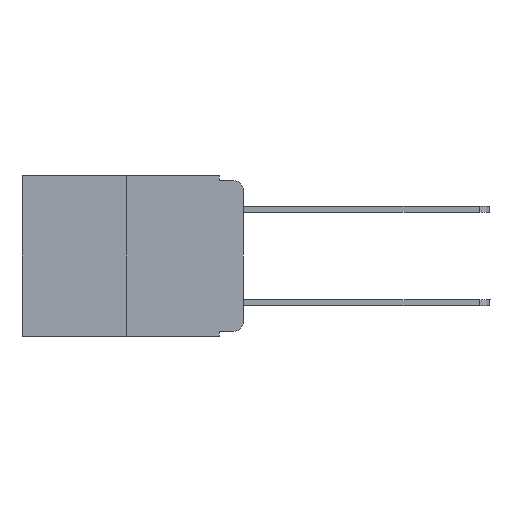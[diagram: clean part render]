
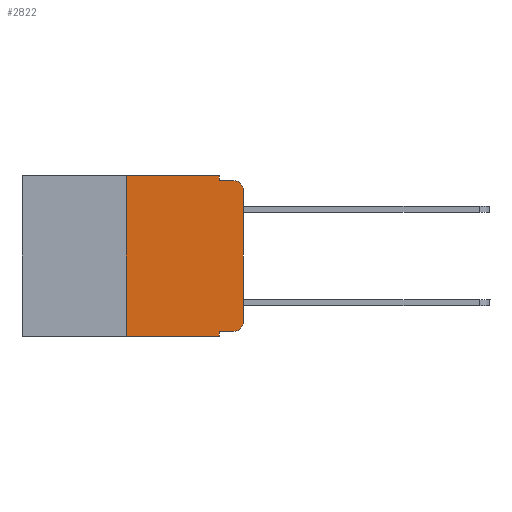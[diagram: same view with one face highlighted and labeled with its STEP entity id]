
A CAD part, left-side view. The second image highlights one B-rep face of the part: STEP entity #2822.
In plain terms, the highlighted planar face has unit normal (-1, 0, 0).
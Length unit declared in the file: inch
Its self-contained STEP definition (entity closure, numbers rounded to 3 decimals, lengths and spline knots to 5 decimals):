
#67 = LINE ( 'NONE', #15647, #533 ) ;
#316 = CARTESIAN_POINT ( 'NONE',  ( 0., 0.473, 0. ) ) ;
#466 = VECTOR ( 'NONE', #7113, 39.37008 ) ;
#524 = CARTESIAN_POINT ( 'NONE',  ( 0., 0.473, 0. ) ) ;
#533 = VECTOR ( 'NONE', #4068, 39.37008 ) ;
#613 = VECTOR ( 'NONE', #11572, 39.37008 ) ;
#622 = LINE ( 'NONE', #12232, #9896 ) ;
#713 = ORIENTED_EDGE ( 'NONE', *, *, #8931, .F. ) ;
#740 = ORIENTED_EDGE ( 'NONE', *, *, #4380, .T. ) ;
#883 = CARTESIAN_POINT ( 'NONE',  ( 0., 0.25, -0.343 ) ) ;
#1070 = CIRCLE ( 'NONE', #5091, 0.02 ) ;
#1348 = EDGE_CURVE ( 'NONE', #3318, #15145, #14514, .T. ) ;
#1510 = VERTEX_POINT ( 'NONE', #8373 ) ;
#2126 = VERTEX_POINT ( 'NONE', #2161 ) ;
#2161 = CARTESIAN_POINT ( 'NONE',  ( 0., 0., -0.313 ) ) ;
#2480 = EDGE_CURVE ( 'NONE', #13575, #7105, #11095, .T. ) ;
#2576 = DIRECTION ( 'NONE',  ( 0., 0., -1. ) ) ;
#2800 = CARTESIAN_POINT ( 'NONE',  ( 0., 0., 0. ) ) ;
#2822 = ADVANCED_FACE ( 'NONE', ( #15793 ), #3281, .F. ) ;
#3091 = DIRECTION ( 'NONE',  ( 0., 0., -1. ) ) ;
#3263 = ORIENTED_EDGE ( 'NONE', *, *, #14166, .F. ) ;
#3281 = PLANE ( 'NONE',  #10324 ) ;
#3283 = DIRECTION ( 'NONE',  ( 0., 0., -1. ) ) ;
#3318 = VERTEX_POINT ( 'NONE', #14580 ) ;
#3766 = EDGE_LOOP ( 'NONE', ( #4187, #4413, #16521, #8316, #713, #3263, #740, #11215, #14098, #5282 ) ) ;
#3894 = CARTESIAN_POINT ( 'NONE',  ( 0., 0.051, -0.333 ) ) ;
#4068 = DIRECTION ( 'NONE',  ( 0., -1., 0. ) ) ;
#4187 = ORIENTED_EDGE ( 'NONE', *, *, #14029, .T. ) ;
#4380 = EDGE_CURVE ( 'NONE', #9209, #7105, #622, .T. ) ;
#4413 = ORIENTED_EDGE ( 'NONE', *, *, #1348, .T. ) ;
#5091 = AXIS2_PLACEMENT_3D ( 'NONE', #11053, #14840, #3283 ) ;
#5282 = ORIENTED_EDGE ( 'NONE', *, *, #15119, .T. ) ;
#5348 = VERTEX_POINT ( 'NONE', #8810 ) ;
#6153 = DIRECTION ( 'NONE',  ( 0., -1., 0. ) ) ;
#6494 = LINE ( 'NONE', #2800, #613 ) ;
#6747 = DIRECTION ( 'NONE',  ( 1., 0., 0. ) ) ;
#7105 = VERTEX_POINT ( 'NONE', #16439 ) ;
#7113 = DIRECTION ( 'NONE',  ( 0., -1., 0. ) ) ;
#7128 = VECTOR ( 'NONE', #9408, 39.37008 ) ;
#7238 = AXIS2_PLACEMENT_3D ( 'NONE', #10264, #14118, #2576 ) ;
#7342 = EDGE_CURVE ( 'NONE', #13575, #9813, #11015, .T. ) ;
#8316 = ORIENTED_EDGE ( 'NONE', *, *, #10362, .F. ) ;
#8373 = CARTESIAN_POINT ( 'NONE',  ( 0., 0.25, 0. ) ) ;
#8472 = CARTESIAN_POINT ( 'NONE',  ( 0., 0.02, -0.333 ) ) ;
#8810 = CARTESIAN_POINT ( 'NONE',  ( 0., 0.051, 0. ) ) ;
#8931 = EDGE_CURVE ( 'NONE', #1510, #5348, #15664, .T. ) ;
#9209 = VERTEX_POINT ( 'NONE', #883 ) ;
#9408 = DIRECTION ( 'NONE',  ( 0., -1., 0. ) ) ;
#9813 = VERTEX_POINT ( 'NONE', #8472 ) ;
#9896 = VECTOR ( 'NONE', #6153, 39.37008 ) ;
#10043 = VECTOR ( 'NONE', #10732, 39.37008 ) ;
#10264 = CARTESIAN_POINT ( 'NONE',  ( 0., 0.02, -0.03 ) ) ;
#10324 = AXIS2_PLACEMENT_3D ( 'NONE', #524, #6747, #10811 ) ;
#10362 = EDGE_CURVE ( 'NONE', #5348, #15535, #13296, .T. ) ;
#10645 = LINE ( 'NONE', #13476, #10043 ) ;
#10732 = DIRECTION ( 'NONE',  ( 0., 0., 1. ) ) ;
#10811 = DIRECTION ( 'NONE',  ( 0., 0., -1. ) ) ;
#10991 = EDGE_CURVE ( 'NONE', #15535, #15145, #67, .T. ) ;
#11015 = LINE ( 'NONE', #13288, #466 ) ;
#11053 = CARTESIAN_POINT ( 'NONE',  ( 0., 0.02, -0.313 ) ) ;
#11095 = LINE ( 'NONE', #16235, #11997 ) ;
#11215 = ORIENTED_EDGE ( 'NONE', *, *, #2480, .F. ) ;
#11572 = DIRECTION ( 'NONE',  ( 0., 0., 1. ) ) ;
#11997 = VECTOR ( 'NONE', #14792, 39.37008 ) ;
#12232 = CARTESIAN_POINT ( 'NONE',  ( 0., 0.473, -0.343 ) ) ;
#13288 = CARTESIAN_POINT ( 'NONE',  ( 0., 0.051, -0.333 ) ) ;
#13296 = LINE ( 'NONE', #15937, #14258 ) ;
#13462 = CARTESIAN_POINT ( 'NONE',  ( 0., 0.051, -0.01 ) ) ;
#13476 = CARTESIAN_POINT ( 'NONE',  ( 0., 0.25, 0. ) ) ;
#13575 = VERTEX_POINT ( 'NONE', #3894 ) ;
#14029 = EDGE_CURVE ( 'NONE', #2126, #3318, #6494, .T. ) ;
#14098 = ORIENTED_EDGE ( 'NONE', *, *, #7342, .T. ) ;
#14118 = DIRECTION ( 'NONE',  ( -1., 0., 0. ) ) ;
#14166 = EDGE_CURVE ( 'NONE', #9209, #1510, #10645, .T. ) ;
#14258 = VECTOR ( 'NONE', #3091, 39.37008 ) ;
#14514 = CIRCLE ( 'NONE', #7238, 0.02 ) ;
#14580 = CARTESIAN_POINT ( 'NONE',  ( 0., 0., -0.03 ) ) ;
#14792 = DIRECTION ( 'NONE',  ( 0., 0., -1. ) ) ;
#14840 = DIRECTION ( 'NONE',  ( -1., 0., 0. ) ) ;
#15119 = EDGE_CURVE ( 'NONE', #9813, #2126, #1070, .T. ) ;
#15145 = VERTEX_POINT ( 'NONE', #16546 ) ;
#15535 = VERTEX_POINT ( 'NONE', #13462 ) ;
#15647 = CARTESIAN_POINT ( 'NONE',  ( 0., 0.051, -0.01 ) ) ;
#15664 = LINE ( 'NONE', #316, #7128 ) ;
#15793 = FACE_OUTER_BOUND ( 'NONE', #3766, .T. ) ;
#15937 = CARTESIAN_POINT ( 'NONE',  ( 0., 0.051, 0. ) ) ;
#16235 = CARTESIAN_POINT ( 'NONE',  ( 0., 0.051, 0. ) ) ;
#16439 = CARTESIAN_POINT ( 'NONE',  ( 0., 0.051, -0.343 ) ) ;
#16521 = ORIENTED_EDGE ( 'NONE', *, *, #10991, .F. ) ;
#16546 = CARTESIAN_POINT ( 'NONE',  ( 0., 0.02, -0.01 ) ) ;
